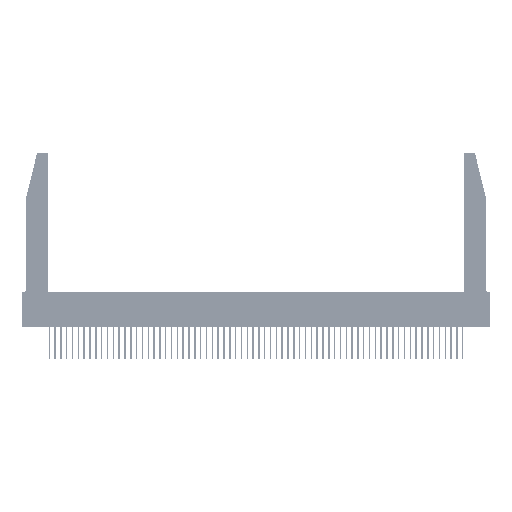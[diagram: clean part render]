
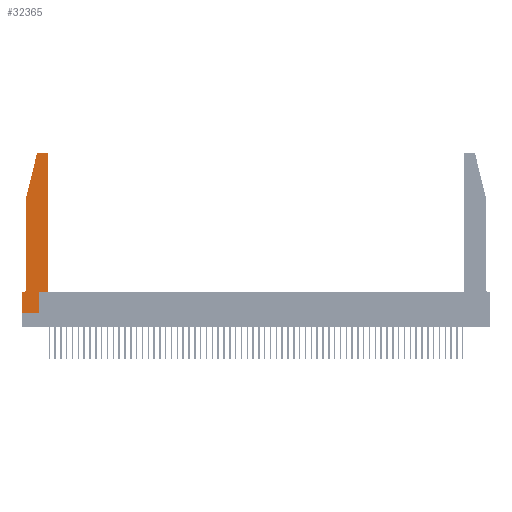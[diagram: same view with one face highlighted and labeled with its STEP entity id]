
A CAD part, top view. The second image highlights one B-rep face of the part: STEP entity #32365.
In plain terms, the highlighted planar face has unit normal (0, 0, 1).
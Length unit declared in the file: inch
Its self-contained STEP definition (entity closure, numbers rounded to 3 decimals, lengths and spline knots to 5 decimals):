
#184 = EDGE_CURVE ( 'NONE', #28665, #30767, #19172, .T. ) ;
#1346 = CARTESIAN_POINT ( 'NONE',  ( 0.4505, 0.35, 0.37 ) ) ;
#2221 = CARTESIAN_POINT ( 'NONE',  ( 0.4205, 2.72, 0.37 ) ) ;
#2604 = DIRECTION ( 'NONE',  ( -1., 0., 0. ) ) ;
#3310 = CARTESIAN_POINT ( 'NONE',  ( 0.2865, 0.35, 0.37 ) ) ;
#3416 = CARTESIAN_POINT ( 'NONE',  ( 0.0755, 0.42, 0.37 ) ) ;
#3642 = VERTEX_POINT ( 'NONE', #25091 ) ;
#3861 = CARTESIAN_POINT ( 'NONE',  ( 0.0755, 0.35, 0.37 ) ) ;
#4672 = DIRECTION ( 'NONE',  ( 0., 0., -1. ) ) ;
#4981 = LINE ( 'NONE', #34165, #27262 ) ;
#5381 = CARTESIAN_POINT ( 'NONE',  ( 0.25487, 2.72718, 0.37 ) ) ;
#5886 = DIRECTION ( 'NONE',  ( 0., 1., 0. ) ) ;
#6545 = AXIS2_PLACEMENT_3D ( 'NONE', #31282, #4672, #35725 ) ;
#6609 = VECTOR ( 'NONE', #34931, 39.37008 ) ;
#6736 = DIRECTION ( 'NONE',  ( 1., 0., 0. ) ) ;
#8019 = LINE ( 'NONE', #3861, #6609 ) ;
#8756 = ORIENTED_EDGE ( 'NONE', *, *, #184, .T. ) ;
#9153 = VERTEX_POINT ( 'NONE', #48355 ) ;
#9311 = LINE ( 'NONE', #10801, #31517 ) ;
#9397 = PLANE ( 'NONE',  #41300 ) ;
#10445 = FACE_OUTER_BOUND ( 'NONE', #50075, .T. ) ;
#10742 = EDGE_CURVE ( 'NONE', #36980, #3642, #28693, .T. ) ;
#10801 = CARTESIAN_POINT ( 'NONE',  ( 0.0755, 2., 0.37 ) ) ;
#11933 = EDGE_CURVE ( 'NONE', #30767, #13742, #4981, .T. ) ;
#12338 = VERTEX_POINT ( 'NONE', #5381 ) ;
#13742 = VERTEX_POINT ( 'NONE', #37638 ) ;
#15319 = DIRECTION ( 'NONE',  ( 0., -1., 0. ) ) ;
#16943 = LINE ( 'NONE', #47505, #50654 ) ;
#17355 = AXIS2_PLACEMENT_3D ( 'NONE', #2221, #33331, #6736 ) ;
#17546 = EDGE_CURVE ( 'NONE', #12338, #9153, #31413, .T. ) ;
#17805 = VECTOR ( 'NONE', #50507, 39.37008 ) ;
#18321 = VECTOR ( 'NONE', #2604, 39.37008 ) ;
#18373 = DIRECTION ( 'NONE',  ( 0., 0., 1. ) ) ;
#19172 = LINE ( 'NONE', #19744, #17805 ) ;
#19670 = CARTESIAN_POINT ( 'NONE',  ( 0., 0.35, 0.37 ) ) ;
#19702 = DIRECTION ( 'NONE',  ( -0.239, -0.971, 0. ) ) ;
#19744 = CARTESIAN_POINT ( 'NONE',  ( 0., 0., 0.37 ) ) ;
#21059 = VECTOR ( 'NONE', #19702, 39.37008 ) ;
#21496 = EDGE_CURVE ( 'NONE', #9153, #24941, #9311, .T. ) ;
#22950 = EDGE_CURVE ( 'NONE', #39119, #41403, #38292, .T. ) ;
#23069 = CARTESIAN_POINT ( 'NONE',  ( 0.4505, 2.72, 0.37 ) ) ;
#23828 = CARTESIAN_POINT ( 'NONE',  ( 0.4205, 2.75, 0.37 ) ) ;
#24941 = VERTEX_POINT ( 'NONE', #3416 ) ;
#25091 = CARTESIAN_POINT ( 'NONE',  ( 0.284, 2.75, 0.37 ) ) ;
#26167 = DIRECTION ( 'NONE',  ( 0., 0., 1. ) ) ;
#26618 = VECTOR ( 'NONE', #55696, 39.37008 ) ;
#27262 = VECTOR ( 'NONE', #38556, 39.37008 ) ;
#28665 = VERTEX_POINT ( 'NONE', #19670 ) ;
#28693 = LINE ( 'NONE', #37916, #18321 ) ;
#28964 = CARTESIAN_POINT ( 'NONE',  ( 0., 0., 0.37 ) ) ;
#29274 = CARTESIAN_POINT ( 'NONE',  ( 0.4505, 0.35, 0.37 ) ) ;
#29541 = AXIS2_PLACEMENT_3D ( 'NONE', #52451, #26167, #56826 ) ;
#29687 = ORIENTED_EDGE ( 'NONE', *, *, #41654, .T. ) ;
#30724 = CIRCLE ( 'NONE', #6545, 0.07 ) ;
#30767 = VERTEX_POINT ( 'NONE', #28964 ) ;
#31282 = CARTESIAN_POINT ( 'NONE',  ( 0.0055, 0.42, 0.37 ) ) ;
#31413 = LINE ( 'NONE', #46063, #21059 ) ;
#31517 = VECTOR ( 'NONE', #15319, 39.37008 ) ;
#31790 = ORIENTED_EDGE ( 'NONE', *, *, #38551, .T. ) ;
#32365 = ADVANCED_FACE ( 'NONE', ( #10445 ), #9397, .T. ) ;
#32443 = ORIENTED_EDGE ( 'NONE', *, *, #10742, .T. ) ;
#32455 = LINE ( 'NONE', #1346, #54373 ) ;
#33319 = EDGE_CURVE ( 'NONE', #48717, #36980, #54454, .T. ) ;
#33331 = DIRECTION ( 'NONE',  ( 0., 0., 1. ) ) ;
#34165 = CARTESIAN_POINT ( 'NONE',  ( 0., 0., 0.37 ) ) ;
#34401 = ORIENTED_EDGE ( 'NONE', *, *, #43513, .T. ) ;
#34931 = DIRECTION ( 'NONE',  ( -1., 0., 0. ) ) ;
#35611 = VERTEX_POINT ( 'NONE', #42162 ) ;
#35725 = DIRECTION ( 'NONE',  ( -1., 0., 0. ) ) ;
#35890 = ORIENTED_EDGE ( 'NONE', *, *, #22950, .T. ) ;
#36980 = VERTEX_POINT ( 'NONE', #23828 ) ;
#37337 = CIRCLE ( 'NONE', #29541, 0.03 ) ;
#37638 = CARTESIAN_POINT ( 'NONE',  ( 0.2865, 0., 0.37 ) ) ;
#37916 = CARTESIAN_POINT ( 'NONE',  ( 0.2605, 2.75, 0.37 ) ) ;
#38292 = LINE ( 'NONE', #29274, #26618 ) ;
#38544 = ORIENTED_EDGE ( 'NONE', *, *, #33319, .T. ) ;
#38551 = EDGE_CURVE ( 'NONE', #13742, #39119, #16943, .T. ) ;
#38556 = DIRECTION ( 'NONE',  ( 1., 0., 0. ) ) ;
#39119 = VERTEX_POINT ( 'NONE', #3310 ) ;
#41300 = AXIS2_PLACEMENT_3D ( 'NONE', #44726, #18373, #49153 ) ;
#41403 = VERTEX_POINT ( 'NONE', #43848 ) ;
#41654 = EDGE_CURVE ( 'NONE', #41403, #48717, #32455, .T. ) ;
#42162 = CARTESIAN_POINT ( 'NONE',  ( 0.0055, 0.35, 0.37 ) ) ;
#43074 = DIRECTION ( 'NONE',  ( 0., 1., 0. ) ) ;
#43513 = EDGE_CURVE ( 'NONE', #35611, #28665, #8019, .T. ) ;
#43848 = CARTESIAN_POINT ( 'NONE',  ( 0.4505, 0.35, 0.37 ) ) ;
#44726 = CARTESIAN_POINT ( 'NONE',  ( 0., 0.35, 0.37 ) ) ;
#46063 = CARTESIAN_POINT ( 'NONE',  ( 0.0755, 2., 0.37 ) ) ;
#47447 = EDGE_CURVE ( 'NONE', #24941, #35611, #30724, .T. ) ;
#47505 = CARTESIAN_POINT ( 'NONE',  ( 0.2865, 0.35, 0.37 ) ) ;
#48355 = CARTESIAN_POINT ( 'NONE',  ( 0.0755, 2., 0.37 ) ) ;
#48717 = VERTEX_POINT ( 'NONE', #23069 ) ;
#49153 = DIRECTION ( 'NONE',  ( 1., 0., 0. ) ) ;
#50075 = EDGE_LOOP ( 'NONE', ( #32443, #51095, #54865, #56958, #52207, #34401, #8756, #55629, #31790, #35890, #29687, #38544 ) ) ;
#50507 = DIRECTION ( 'NONE',  ( 0., -1., 0. ) ) ;
#50654 = VECTOR ( 'NONE', #43074, 39.37008 ) ;
#51095 = ORIENTED_EDGE ( 'NONE', *, *, #54723, .T. ) ;
#52207 = ORIENTED_EDGE ( 'NONE', *, *, #47447, .T. ) ;
#52451 = CARTESIAN_POINT ( 'NONE',  ( 0.284, 2.72, 0.37 ) ) ;
#54373 = VECTOR ( 'NONE', #5886, 39.37008 ) ;
#54454 = CIRCLE ( 'NONE', #17355, 0.03 ) ;
#54723 = EDGE_CURVE ( 'NONE', #3642, #12338, #37337, .T. ) ;
#54865 = ORIENTED_EDGE ( 'NONE', *, *, #17546, .T. ) ;
#55629 = ORIENTED_EDGE ( 'NONE', *, *, #11933, .T. ) ;
#55696 = DIRECTION ( 'NONE',  ( 1., 0., 0. ) ) ;
#56826 = DIRECTION ( 'NONE',  ( 1., 0., 0. ) ) ;
#56958 = ORIENTED_EDGE ( 'NONE', *, *, #21496, .T. ) ;
